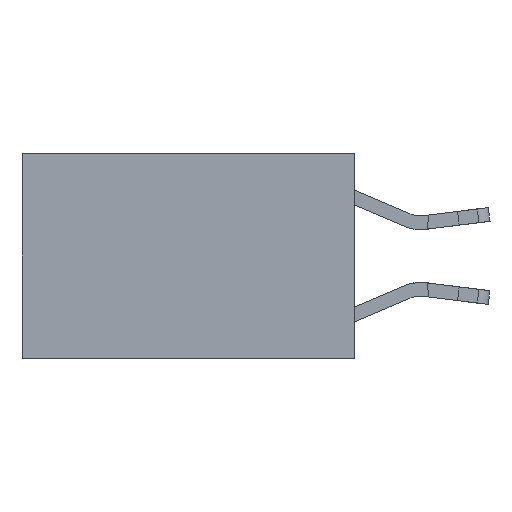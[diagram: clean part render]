
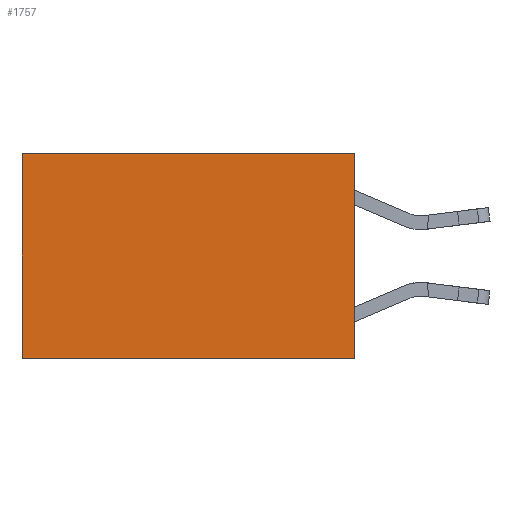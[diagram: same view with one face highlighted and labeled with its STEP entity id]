
A CAD part, left-side view. The second image highlights one B-rep face of the part: STEP entity #1757.
In plain terms, the highlighted planar face has unit normal (-1, 0, 0).
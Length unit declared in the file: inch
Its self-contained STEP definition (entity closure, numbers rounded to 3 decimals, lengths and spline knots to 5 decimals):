
#80 = LINE ( 'NONE', #6688, #27176 ) ;
#474 = EDGE_CURVE ( 'NONE', #24193, #8490, #6670, .T. ) ;
#503 = ORIENTED_EDGE ( 'NONE', *, *, #11431, .F. ) ;
#1121 = DIRECTION ( 'NONE',  ( 0., 0., -1. ) ) ;
#1757 = ADVANCED_FACE ( 'NONE', ( #17490 ), #14939, .F. ) ;
#1945 = CARTESIAN_POINT ( 'NONE',  ( 0.2625, 0., 0. ) ) ;
#4392 = EDGE_CURVE ( 'NONE', #21631, #9073, #17419, .T. ) ;
#5424 = DIRECTION ( 'NONE',  ( 0., 1., 0. ) ) ;
#5434 = CARTESIAN_POINT ( 'NONE',  ( 0.2625, 0., 0. ) ) ;
#6018 = CARTESIAN_POINT ( 'NONE',  ( 0.2625, 0., -0.37 ) ) ;
#6030 = EDGE_CURVE ( 'NONE', #21631, #24193, #19049, .T. ) ;
#6670 = LINE ( 'NONE', #27322, #17127 ) ;
#6688 = CARTESIAN_POINT ( 'NONE',  ( 0.2625, 0., -0.37 ) ) ;
#7510 = VECTOR ( 'NONE', #10805, 39.37008 ) ;
#8490 = VERTEX_POINT ( 'NONE', #18533 ) ;
#9073 = VERTEX_POINT ( 'NONE', #6018 ) ;
#9315 = EDGE_LOOP ( 'NONE', ( #22411, #503, #19342, #27893 ) ) ;
#10592 = CARTESIAN_POINT ( 'NONE',  ( 0.2625, 0., 0. ) ) ;
#10805 = DIRECTION ( 'NONE',  ( 0., 0., -1. ) ) ;
#11431 = EDGE_CURVE ( 'NONE', #9073, #8490, #80, .T. ) ;
#12975 = DIRECTION ( 'NONE',  ( 1., 0., 0. ) ) ;
#13878 = AXIS2_PLACEMENT_3D ( 'NONE', #10592, #12975, #1121 ) ;
#14939 = PLANE ( 'NONE',  #13878 ) ;
#16817 = CARTESIAN_POINT ( 'NONE',  ( 0.2625, 0., 0. ) ) ;
#17127 = VECTOR ( 'NONE', #27030, 39.37008 ) ;
#17419 = LINE ( 'NONE', #1945, #7510 ) ;
#17490 = FACE_OUTER_BOUND ( 'NONE', #9315, .T. ) ;
#18238 = CARTESIAN_POINT ( 'NONE',  ( 0.2625, 0.6, 0. ) ) ;
#18533 = CARTESIAN_POINT ( 'NONE',  ( 0.2625, 0.6, -0.37 ) ) ;
#19049 = LINE ( 'NONE', #16817, #27410 ) ;
#19342 = ORIENTED_EDGE ( 'NONE', *, *, #4392, .F. ) ;
#21631 = VERTEX_POINT ( 'NONE', #5434 ) ;
#22411 = ORIENTED_EDGE ( 'NONE', *, *, #474, .T. ) ;
#22577 = DIRECTION ( 'NONE',  ( 0., 1., 0. ) ) ;
#24193 = VERTEX_POINT ( 'NONE', #18238 ) ;
#27030 = DIRECTION ( 'NONE',  ( 0., 0., -1. ) ) ;
#27176 = VECTOR ( 'NONE', #22577, 39.37008 ) ;
#27322 = CARTESIAN_POINT ( 'NONE',  ( 0.2625, 0.6, 0. ) ) ;
#27410 = VECTOR ( 'NONE', #5424, 39.37008 ) ;
#27893 = ORIENTED_EDGE ( 'NONE', *, *, #6030, .T. ) ;
